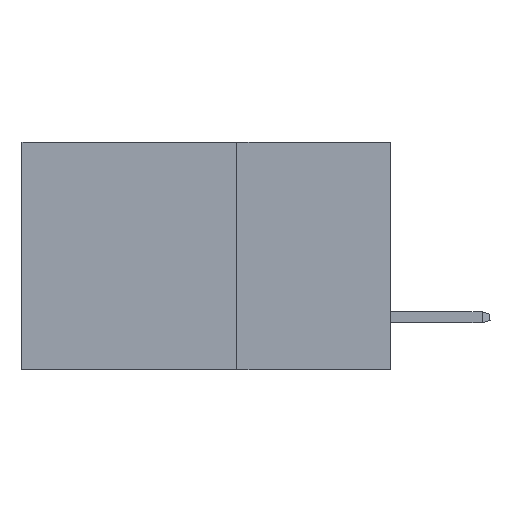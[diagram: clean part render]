
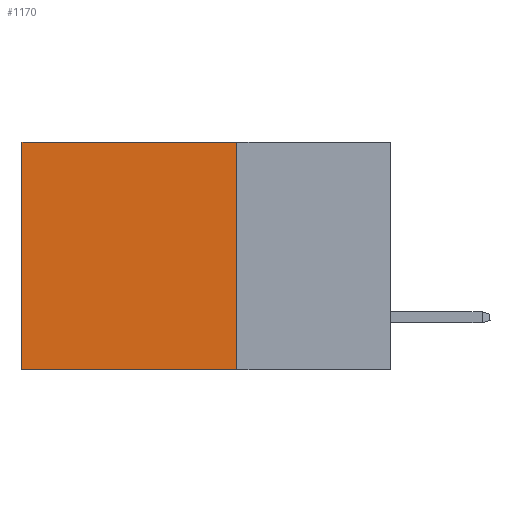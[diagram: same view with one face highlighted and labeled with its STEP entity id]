
A CAD part, left-side view. The second image highlights one B-rep face of the part: STEP entity #1170.
In plain terms, the highlighted planar face has unit normal (-1, 0, 0).
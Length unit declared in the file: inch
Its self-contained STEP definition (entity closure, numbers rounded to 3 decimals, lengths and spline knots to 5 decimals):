
#321 = CARTESIAN_POINT ( 'NONE',  ( 0.2875, 0.25, 0. ) ) ;
#411 = ORIENTED_EDGE ( 'NONE', *, *, #8398, .F. ) ;
#582 = PLANE ( 'NONE',  #17932 ) ;
#593 = VERTEX_POINT ( 'NONE', #7354 ) ;
#850 = FACE_OUTER_BOUND ( 'NONE', #11101, .T. ) ;
#1170 = ADVANCED_FACE ( 'NONE', ( #850 ), #582, .F. ) ;
#2065 = CARTESIAN_POINT ( 'NONE',  ( 0.2875, 0.25, 0. ) ) ;
#2418 = EDGE_CURVE ( 'NONE', #10845, #13770, #19345, .T. ) ;
#4825 = CARTESIAN_POINT ( 'NONE',  ( 0.2875, 0.25, -0.37 ) ) ;
#6196 = ORIENTED_EDGE ( 'NONE', *, *, #2418, .T. ) ;
#7354 = CARTESIAN_POINT ( 'NONE',  ( 0.2875, 0.25, -0.37 ) ) ;
#7675 = VECTOR ( 'NONE', #16276, 39.37008 ) ;
#7686 = CARTESIAN_POINT ( 'NONE',  ( 0.2875, 0.25, 0. ) ) ;
#8398 = EDGE_CURVE ( 'NONE', #593, #15629, #13555, .T. ) ;
#8515 = ORIENTED_EDGE ( 'NONE', *, *, #16845, .T. ) ;
#8820 = EDGE_CURVE ( 'NONE', #10845, #593, #16596, .T. ) ;
#9354 = CARTESIAN_POINT ( 'NONE',  ( 0.2875, 0.6, -0.37 ) ) ;
#9721 = VECTOR ( 'NONE', #11477, 39.37008 ) ;
#10845 = VERTEX_POINT ( 'NONE', #321 ) ;
#11101 = EDGE_LOOP ( 'NONE', ( #8515, #411, #18821, #6196 ) ) ;
#11477 = DIRECTION ( 'NONE',  ( 0., 0., -1. ) ) ;
#11615 = CARTESIAN_POINT ( 'NONE',  ( 0.2875, 0.6, 0. ) ) ;
#12278 = VECTOR ( 'NONE', #16854, 39.37008 ) ;
#13555 = LINE ( 'NONE', #4825, #7675 ) ;
#13612 = CARTESIAN_POINT ( 'NONE',  ( 0.2875, 0.6, 0. ) ) ;
#13770 = VERTEX_POINT ( 'NONE', #13612 ) ;
#15629 = VERTEX_POINT ( 'NONE', #9354 ) ;
#16276 = DIRECTION ( 'NONE',  ( 0., 1., 0. ) ) ;
#16596 = LINE ( 'NONE', #18266, #12278 ) ;
#16845 = EDGE_CURVE ( 'NONE', #13770, #15629, #17132, .T. ) ;
#16854 = DIRECTION ( 'NONE',  ( 0., 0., -1. ) ) ;
#17132 = LINE ( 'NONE', #11615, #9721 ) ;
#17932 = AXIS2_PLACEMENT_3D ( 'NONE', #2065, #18689, #20228 ) ;
#18266 = CARTESIAN_POINT ( 'NONE',  ( 0.2875, 0.25, 0. ) ) ;
#18689 = DIRECTION ( 'NONE',  ( 1., 0., 0. ) ) ;
#18821 = ORIENTED_EDGE ( 'NONE', *, *, #8820, .F. ) ;
#18851 = VECTOR ( 'NONE', #20733, 39.37008 ) ;
#19345 = LINE ( 'NONE', #7686, #18851 ) ;
#20228 = DIRECTION ( 'NONE',  ( 0., 0., -1. ) ) ;
#20733 = DIRECTION ( 'NONE',  ( 0., 1., 0. ) ) ;
